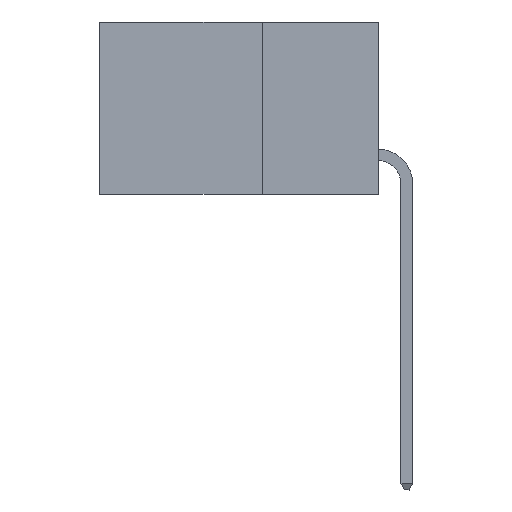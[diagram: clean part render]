
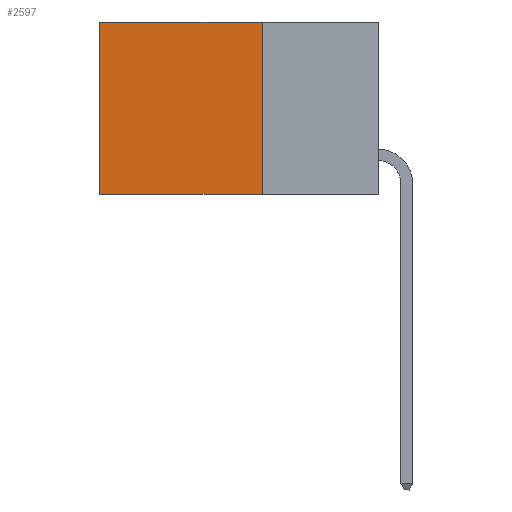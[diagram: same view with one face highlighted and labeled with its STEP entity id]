
A CAD part, left-side view. The second image highlights one B-rep face of the part: STEP entity #2597.
In plain terms, the highlighted planar face has unit normal (-1, 0, 0).
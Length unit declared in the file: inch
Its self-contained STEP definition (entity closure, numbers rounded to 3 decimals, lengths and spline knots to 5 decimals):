
#72 = VECTOR ( 'NONE', #4493, 39.37008 ) ;
#85 = LINE ( 'NONE', #683, #72 ) ;
#298 = VERTEX_POINT ( 'NONE', #11429 ) ;
#316 = LINE ( 'NONE', #5118, #5701 ) ;
#559 = DIRECTION ( 'NONE',  ( 0., 1., 0. ) ) ;
#683 = CARTESIAN_POINT ( 'NONE',  ( 0.298, 0.6, 0. ) ) ;
#1104 = FACE_OUTER_BOUND ( 'NONE', #4468, .T. ) ;
#1694 = CARTESIAN_POINT ( 'NONE',  ( 0.298, 0.25, 0. ) ) ;
#2000 = CARTESIAN_POINT ( 'NONE',  ( 0.298, 0.6, 0. ) ) ;
#2108 = DIRECTION ( 'NONE',  ( 0., 0., -1. ) ) ;
#2130 = LINE ( 'NONE', #4902, #11457 ) ;
#2244 = CARTESIAN_POINT ( 'NONE',  ( 0.298, 0.6, -0.37 ) ) ;
#2443 = EDGE_CURVE ( 'NONE', #10390, #9782, #2130, .T. ) ;
#2597 = ADVANCED_FACE ( 'NONE', ( #1104 ), #2996, .F. ) ;
#2996 = PLANE ( 'NONE',  #6515 ) ;
#3161 = LINE ( 'NONE', #1694, #9909 ) ;
#3930 = CARTESIAN_POINT ( 'NONE',  ( 0.298, 0.25, 0. ) ) ;
#4468 = EDGE_LOOP ( 'NONE', ( #7322, #8881, #9190, #7004 ) ) ;
#4493 = DIRECTION ( 'NONE',  ( 0., 0., -1. ) ) ;
#4902 = CARTESIAN_POINT ( 'NONE',  ( 0.298, 0.25, 0. ) ) ;
#5118 = CARTESIAN_POINT ( 'NONE',  ( 0.298, 0.25, -0.37 ) ) ;
#5701 = VECTOR ( 'NONE', #559, 39.37008 ) ;
#6446 = EDGE_CURVE ( 'NONE', #9782, #6835, #85, .T. ) ;
#6515 = AXIS2_PLACEMENT_3D ( 'NONE', #3930, #10481, #2108 ) ;
#6835 = VERTEX_POINT ( 'NONE', #2244 ) ;
#7004 = ORIENTED_EDGE ( 'NONE', *, *, #2443, .T. ) ;
#7322 = ORIENTED_EDGE ( 'NONE', *, *, #6446, .T. ) ;
#8198 = EDGE_CURVE ( 'NONE', #298, #6835, #316, .T. ) ;
#8881 = ORIENTED_EDGE ( 'NONE', *, *, #8198, .F. ) ;
#9190 = ORIENTED_EDGE ( 'NONE', *, *, #9307, .F. ) ;
#9194 = DIRECTION ( 'NONE',  ( 0., 0., -1. ) ) ;
#9307 = EDGE_CURVE ( 'NONE', #10390, #298, #3161, .T. ) ;
#9401 = CARTESIAN_POINT ( 'NONE',  ( 0.298, 0.25, 0. ) ) ;
#9782 = VERTEX_POINT ( 'NONE', #2000 ) ;
#9909 = VECTOR ( 'NONE', #9194, 39.37008 ) ;
#10390 = VERTEX_POINT ( 'NONE', #9401 ) ;
#10481 = DIRECTION ( 'NONE',  ( 1., 0., 0. ) ) ;
#10584 = DIRECTION ( 'NONE',  ( 0., 1., 0. ) ) ;
#11429 = CARTESIAN_POINT ( 'NONE',  ( 0.298, 0.25, -0.37 ) ) ;
#11457 = VECTOR ( 'NONE', #10584, 39.37008 ) ;
